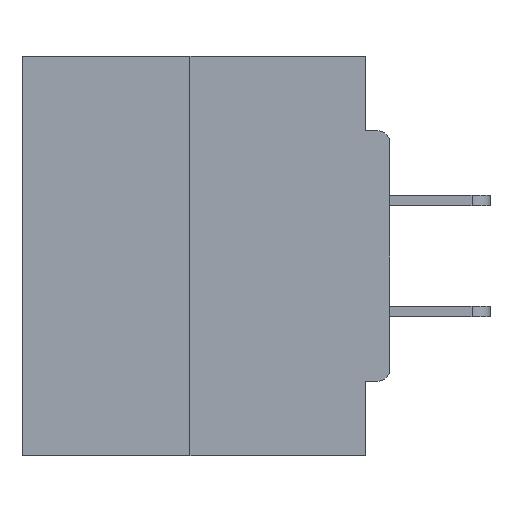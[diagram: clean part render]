
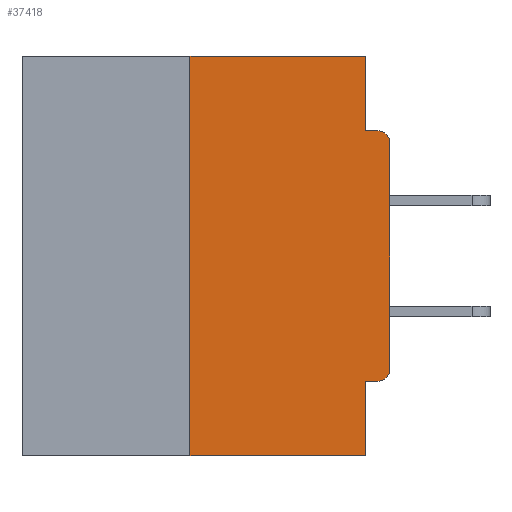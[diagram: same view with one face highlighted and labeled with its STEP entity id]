
A CAD part, left-side view. The second image highlights one B-rep face of the part: STEP entity #37418.
In plain terms, the highlighted planar face has unit normal (-1, 0, 0).
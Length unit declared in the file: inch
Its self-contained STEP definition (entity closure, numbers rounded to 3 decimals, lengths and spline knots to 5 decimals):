
#1209 = DIRECTION ( 'NONE',  ( 0., 0., -1. ) ) ;
#1366 = CARTESIAN_POINT ( 'NONE',  ( 0., 0.015, -0.0935 ) ) ;
#1722 = EDGE_CURVE ( 'NONE', #45793, #41751, #15390, .T. ) ;
#2421 = EDGE_CURVE ( 'NONE', #4091, #23838, #42562, .T. ) ;
#2558 = CARTESIAN_POINT ( 'NONE',  ( 0., 0.015, -0.4065 ) ) ;
#3973 = DIRECTION ( 'NONE',  ( -1., 0., 0. ) ) ;
#4091 = VERTEX_POINT ( 'NONE', #2558 ) ;
#4095 = EDGE_CURVE ( 'NONE', #27829, #43525, #10132, .T. ) ;
#4750 = CARTESIAN_POINT ( 'NONE',  ( 0., 0.46, 0. ) ) ;
#5391 = CIRCLE ( 'NONE', #17557, 0.015 ) ;
#5828 = LINE ( 'NONE', #24205, #11472 ) ;
#5928 = VERTEX_POINT ( 'NONE', #1366 ) ;
#7420 = EDGE_CURVE ( 'NONE', #23838, #16552, #41807, .T. ) ;
#7437 = ORIENTED_EDGE ( 'NONE', *, *, #23754, .F. ) ;
#10132 = LINE ( 'NONE', #13087, #37871 ) ;
#11278 = VECTOR ( 'NONE', #15113, 39.37008 ) ;
#11346 = CARTESIAN_POINT ( 'NONE',  ( 0., 0., -0.4065 ) ) ;
#11472 = VECTOR ( 'NONE', #27690, 39.37008 ) ;
#11979 = DIRECTION ( 'NONE',  ( 1., 0., 0. ) ) ;
#12105 = CIRCLE ( 'NONE', #34933, 0.015 ) ;
#13087 = CARTESIAN_POINT ( 'NONE',  ( 0., 0., 0. ) ) ;
#13650 = AXIS2_PLACEMENT_3D ( 'NONE', #4750, #11979, #44190 ) ;
#13689 = ORIENTED_EDGE ( 'NONE', *, *, #24043, .F. ) ;
#14134 = CARTESIAN_POINT ( 'NONE',  ( 0., 0.031, -0.5 ) ) ;
#15093 = EDGE_LOOP ( 'NONE', ( #42120, #18708, #39316, #43788, #45939, #33338, #32083, #16828, #7437, #13689 ) ) ;
#15113 = DIRECTION ( 'NONE',  ( 0., -1., 0. ) ) ;
#15390 = LINE ( 'NONE', #26154, #45354 ) ;
#16074 = EDGE_CURVE ( 'NONE', #43525, #5928, #5391, .T. ) ;
#16552 = VERTEX_POINT ( 'NONE', #14134 ) ;
#16828 = ORIENTED_EDGE ( 'NONE', *, *, #16074, .T. ) ;
#16849 = VECTOR ( 'NONE', #32887, 39.37008 ) ;
#17557 = AXIS2_PLACEMENT_3D ( 'NONE', #41286, #26129, #30998 ) ;
#18586 = LINE ( 'NONE', #21306, #11278 ) ;
#18708 = ORIENTED_EDGE ( 'NONE', *, *, #1722, .F. ) ;
#19737 = LINE ( 'NONE', #29906, #28207 ) ;
#21306 = CARTESIAN_POINT ( 'NONE',  ( 0., 0., -0.0935 ) ) ;
#21705 = CARTESIAN_POINT ( 'NONE',  ( 0., 0.031, -0.0935 ) ) ;
#22082 = CARTESIAN_POINT ( 'NONE',  ( 0., 0.031, -0.4065 ) ) ;
#22481 = DIRECTION ( 'NONE',  ( 0., 0., 1. ) ) ;
#22755 = CARTESIAN_POINT ( 'NONE',  ( 0., 0.031, -0.5 ) ) ;
#22952 = CARTESIAN_POINT ( 'NONE',  ( 0., 0.25, 0. ) ) ;
#23754 = EDGE_CURVE ( 'NONE', #43230, #5928, #18586, .T. ) ;
#23819 = DIRECTION ( 'NONE',  ( 0., 0., 1. ) ) ;
#23838 = VERTEX_POINT ( 'NONE', #22082 ) ;
#24043 = EDGE_CURVE ( 'NONE', #30078, #43230, #19737, .T. ) ;
#24146 = EDGE_CURVE ( 'NONE', #41751, #30078, #34455, .T. ) ;
#24205 = CARTESIAN_POINT ( 'NONE',  ( 0., 0.46, -0.5 ) ) ;
#26129 = DIRECTION ( 'NONE',  ( -1., 0., 0. ) ) ;
#26154 = CARTESIAN_POINT ( 'NONE',  ( 0., 0.25, 0. ) ) ;
#27690 = DIRECTION ( 'NONE',  ( 0., -1., 0. ) ) ;
#27829 = VERTEX_POINT ( 'NONE', #34176 ) ;
#28207 = VECTOR ( 'NONE', #40629, 39.37008 ) ;
#29066 = CARTESIAN_POINT ( 'NONE',  ( 0., 0.46, 0. ) ) ;
#29189 = DIRECTION ( 'NONE',  ( 0., 1., 0. ) ) ;
#29195 = DIRECTION ( 'NONE',  ( 0., 0., -1. ) ) ;
#29906 = CARTESIAN_POINT ( 'NONE',  ( 0., 0.031, 0. ) ) ;
#30078 = VERTEX_POINT ( 'NONE', #40615 ) ;
#30810 = FACE_OUTER_BOUND ( 'NONE', #15093, .T. ) ;
#30998 = DIRECTION ( 'NONE',  ( 0., 0., -1. ) ) ;
#31436 = EDGE_CURVE ( 'NONE', #45793, #16552, #5828, .T. ) ;
#32083 = ORIENTED_EDGE ( 'NONE', *, *, #4095, .T. ) ;
#32887 = DIRECTION ( 'NONE',  ( 0., -1., 0. ) ) ;
#32983 = VECTOR ( 'NONE', #29189, 39.37008 ) ;
#33338 = ORIENTED_EDGE ( 'NONE', *, *, #37968, .T. ) ;
#34176 = CARTESIAN_POINT ( 'NONE',  ( 0., 0., -0.3915 ) ) ;
#34455 = LINE ( 'NONE', #29066, #16849 ) ;
#34933 = AXIS2_PLACEMENT_3D ( 'NONE', #36483, #3973, #29195 ) ;
#36483 = CARTESIAN_POINT ( 'NONE',  ( 0., 0.015, -0.3915 ) ) ;
#37132 = PLANE ( 'NONE',  #13650 ) ;
#37302 = VECTOR ( 'NONE', #1209, 39.37008 ) ;
#37418 = ADVANCED_FACE ( 'NONE', ( #30810 ), #37132, .F. ) ;
#37871 = VECTOR ( 'NONE', #23819, 39.37008 ) ;
#37968 = EDGE_CURVE ( 'NONE', #4091, #27829, #12105, .T. ) ;
#39316 = ORIENTED_EDGE ( 'NONE', *, *, #31436, .T. ) ;
#39513 = CARTESIAN_POINT ( 'NONE',  ( 0., 0., -0.1085 ) ) ;
#40615 = CARTESIAN_POINT ( 'NONE',  ( 0., 0.031, 0. ) ) ;
#40629 = DIRECTION ( 'NONE',  ( 0., 0., -1. ) ) ;
#41286 = CARTESIAN_POINT ( 'NONE',  ( 0., 0.015, -0.1085 ) ) ;
#41751 = VERTEX_POINT ( 'NONE', #22952 ) ;
#41807 = LINE ( 'NONE', #22755, #37302 ) ;
#42120 = ORIENTED_EDGE ( 'NONE', *, *, #24146, .F. ) ;
#42562 = LINE ( 'NONE', #11346, #32983 ) ;
#43230 = VERTEX_POINT ( 'NONE', #21705 ) ;
#43525 = VERTEX_POINT ( 'NONE', #39513 ) ;
#43635 = CARTESIAN_POINT ( 'NONE',  ( 0., 0.25, -0.5 ) ) ;
#43788 = ORIENTED_EDGE ( 'NONE', *, *, #7420, .F. ) ;
#44190 = DIRECTION ( 'NONE',  ( 0., 0., -1. ) ) ;
#45354 = VECTOR ( 'NONE', #22481, 39.37008 ) ;
#45793 = VERTEX_POINT ( 'NONE', #43635 ) ;
#45939 = ORIENTED_EDGE ( 'NONE', *, *, #2421, .F. ) ;
